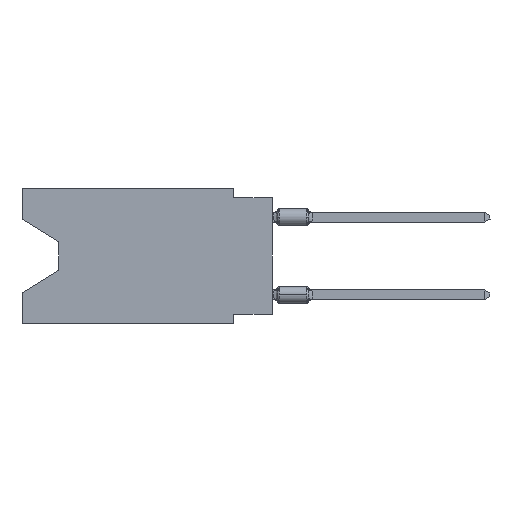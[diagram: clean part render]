
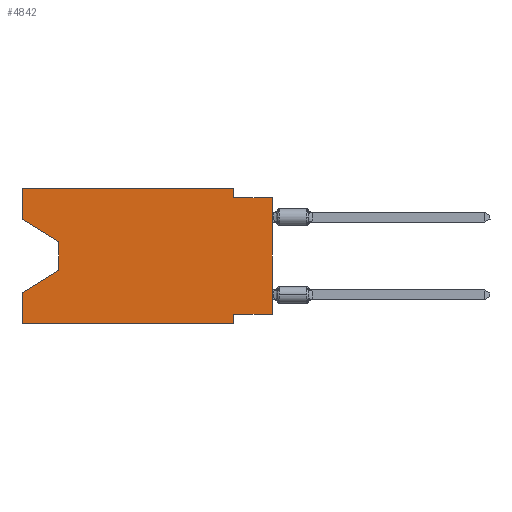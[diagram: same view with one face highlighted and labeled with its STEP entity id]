
A CAD part, left-side view. The second image highlights one B-rep face of the part: STEP entity #4842.
In plain terms, the highlighted planar face has unit normal (-1, 0, 0).
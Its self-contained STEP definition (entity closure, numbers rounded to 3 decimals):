
#241 = CARTESIAN_POINT ( 'NONE',  ( 0., 13.97, -3.505 ) ) ;
#1498 = EDGE_CURVE ( 'NONE', #16888, #11279, #6890, .T. ) ;
#1692 = DIRECTION ( 'NONE',  ( 0., 0., 1. ) ) ;
#2152 = VECTOR ( 'NONE', #27489, 1000. ) ;
#2357 = FACE_OUTER_BOUND ( 'NONE', #19299, .T. ) ;
#2875 = EDGE_CURVE ( 'NONE', #22233, #11279, #8806, .T. ) ;
#3012 = CARTESIAN_POINT ( 'NONE',  ( 0., 2.54, 0. ) ) ;
#3513 = VERTEX_POINT ( 'NONE', #21518 ) ;
#3789 = CARTESIAN_POINT ( 'NONE',  ( 0., 16.383, 0. ) ) ;
#3862 = EDGE_CURVE ( 'NONE', #16888, #35557, #32718, .T. ) ;
#3987 = DIRECTION ( 'NONE',  ( 0., 0., 1. ) ) ;
#4747 = ORIENTED_EDGE ( 'NONE', *, *, #31451, .F. ) ;
#4842 = ADVANCED_FACE ( 'NONE', ( #2357 ), #22465, .F. ) ;
#4987 = ORIENTED_EDGE ( 'NONE', *, *, #8516, .F. ) ;
#5757 = CARTESIAN_POINT ( 'NONE',  ( 0., 13.97, -3.505 ) ) ;
#6108 = DIRECTION ( 'NONE',  ( 0., 0., -1. ) ) ;
#6248 = EDGE_CURVE ( 'NONE', #24653, #28979, #10407, .T. ) ;
#6860 = ORIENTED_EDGE ( 'NONE', *, *, #25004, .T. ) ;
#6890 = LINE ( 'NONE', #21964, #22662 ) ;
#7233 = CARTESIAN_POINT ( 'NONE',  ( 0., 0., -0.635 ) ) ;
#8295 = LINE ( 'NONE', #31710, #23597 ) ;
#8516 = EDGE_CURVE ( 'NONE', #23268, #36215, #9499, .T. ) ;
#8806 = LINE ( 'NONE', #22407, #21508 ) ;
#9112 = ORIENTED_EDGE ( 'NONE', *, *, #30704, .F. ) ;
#9477 = DIRECTION ( 'NONE',  ( 0., 1., 0. ) ) ;
#9499 = LINE ( 'NONE', #21122, #2152 ) ;
#10407 = LINE ( 'NONE', #16976, #26755 ) ;
#10529 = EDGE_CURVE ( 'NONE', #18770, #3513, #32265, .T. ) ;
#10839 = LINE ( 'NONE', #26115, #38145 ) ;
#11279 = VERTEX_POINT ( 'NONE', #7233 ) ;
#12100 = CARTESIAN_POINT ( 'NONE',  ( 0., 16.383, -8.89 ) ) ;
#12760 = CARTESIAN_POINT ( 'NONE',  ( 0., 2.54, 0. ) ) ;
#13883 = CARTESIAN_POINT ( 'NONE',  ( 0., 13.97, -5.385 ) ) ;
#14752 = AXIS2_PLACEMENT_3D ( 'NONE', #16874, #34483, #29233 ) ;
#14763 = CARTESIAN_POINT ( 'NONE',  ( 0., 16.383, -6.852 ) ) ;
#15538 = ORIENTED_EDGE ( 'NONE', *, *, #6248, .F. ) ;
#16063 = ORIENTED_EDGE ( 'NONE', *, *, #3862, .F. ) ;
#16257 = VECTOR ( 'NONE', #28781, 1000. ) ;
#16424 = DIRECTION ( 'NONE',  ( 0., -1., 0. ) ) ;
#16785 = LINE ( 'NONE', #28576, #37239 ) ;
#16874 = CARTESIAN_POINT ( 'NONE',  ( 0., 16.383, 0. ) ) ;
#16888 = VERTEX_POINT ( 'NONE', #37113 ) ;
#16976 = CARTESIAN_POINT ( 'NONE',  ( 0., 16.383, 0. ) ) ;
#17051 = ORIENTED_EDGE ( 'NONE', *, *, #1498, .T. ) ;
#17569 = DIRECTION ( 'NONE',  ( 0., 0., -1. ) ) ;
#17854 = ORIENTED_EDGE ( 'NONE', *, *, #26642, .T. ) ;
#18095 = CARTESIAN_POINT ( 'NONE',  ( 0., 16.383, -2.038 ) ) ;
#18310 = ORIENTED_EDGE ( 'NONE', *, *, #29201, .T. ) ;
#18395 = VECTOR ( 'NONE', #9477, 1000. ) ;
#18770 = VERTEX_POINT ( 'NONE', #241 ) ;
#19299 = EDGE_LOOP ( 'NONE', ( #6860, #29325, #17854, #15538, #18310, #4747, #16063, #17051, #35981, #9112, #4987, #27794 ) ) ;
#21122 = CARTESIAN_POINT ( 'NONE',  ( 0., 16.383, 0. ) ) ;
#21472 = VERTEX_POINT ( 'NONE', #29192 ) ;
#21508 = VECTOR ( 'NONE', #16424, 1000. ) ;
#21518 = CARTESIAN_POINT ( 'NONE',  ( 0., 13.97, -5.385 ) ) ;
#21730 = EDGE_CURVE ( 'NONE', #37658, #23268, #16785, .T. ) ;
#21964 = CARTESIAN_POINT ( 'NONE',  ( 0., 0., 0. ) ) ;
#22233 = VERTEX_POINT ( 'NONE', #23081 ) ;
#22407 = CARTESIAN_POINT ( 'NONE',  ( 0., 0., -0.635 ) ) ;
#22430 = DIRECTION ( 'NONE',  ( 0., -0.855, -0.519 ) ) ;
#22465 = PLANE ( 'NONE',  #14752 ) ;
#22662 = VECTOR ( 'NONE', #3987, 1000. ) ;
#23081 = CARTESIAN_POINT ( 'NONE',  ( 0., 2.54, -0.635 ) ) ;
#23268 = VERTEX_POINT ( 'NONE', #3789 ) ;
#23597 = VECTOR ( 'NONE', #22430, 1000. ) ;
#24364 = LINE ( 'NONE', #12760, #31333 ) ;
#24653 = VERTEX_POINT ( 'NONE', #12100 ) ;
#25004 = EDGE_CURVE ( 'NONE', #37658, #18770, #8295, .T. ) ;
#26115 = CARTESIAN_POINT ( 'NONE',  ( 0., 16.383, -8.89 ) ) ;
#26642 = EDGE_CURVE ( 'NONE', #3513, #28979, #37125, .T. ) ;
#26755 = VECTOR ( 'NONE', #37302, 1000. ) ;
#27140 = CARTESIAN_POINT ( 'NONE',  ( 0., 2.54, -8.255 ) ) ;
#27489 = DIRECTION ( 'NONE',  ( 0., -1., 0. ) ) ;
#27794 = ORIENTED_EDGE ( 'NONE', *, *, #21730, .F. ) ;
#28576 = CARTESIAN_POINT ( 'NONE',  ( 0., 16.383, 0. ) ) ;
#28781 = DIRECTION ( 'NONE',  ( 0., 0.855, -0.519 ) ) ;
#28979 = VERTEX_POINT ( 'NONE', #14763 ) ;
#29084 = VECTOR ( 'NONE', #17569, 1000. ) ;
#29192 = CARTESIAN_POINT ( 'NONE',  ( 0., 2.54, -8.89 ) ) ;
#29201 = EDGE_CURVE ( 'NONE', #24653, #21472, #10839, .T. ) ;
#29233 = DIRECTION ( 'NONE',  ( 0., 0., -1. ) ) ;
#29325 = ORIENTED_EDGE ( 'NONE', *, *, #10529, .T. ) ;
#30119 = VECTOR ( 'NONE', #6108, 1000. ) ;
#30704 = EDGE_CURVE ( 'NONE', #36215, #22233, #24364, .T. ) ;
#30941 = DIRECTION ( 'NONE',  ( 0., 0., -1. ) ) ;
#31333 = VECTOR ( 'NONE', #30941, 1000. ) ;
#31451 = EDGE_CURVE ( 'NONE', #35557, #21472, #37854, .T. ) ;
#31710 = CARTESIAN_POINT ( 'NONE',  ( 0., 16.383, -2.038 ) ) ;
#32265 = LINE ( 'NONE', #5757, #29084 ) ;
#32318 = CARTESIAN_POINT ( 'NONE',  ( 0., 0., -8.255 ) ) ;
#32718 = LINE ( 'NONE', #32318, #18395 ) ;
#34463 = DIRECTION ( 'NONE',  ( 0., -1., 0. ) ) ;
#34483 = DIRECTION ( 'NONE',  ( 1., 0., 0. ) ) ;
#34947 = CARTESIAN_POINT ( 'NONE',  ( 0., 2.54, -8.89 ) ) ;
#35557 = VERTEX_POINT ( 'NONE', #27140 ) ;
#35981 = ORIENTED_EDGE ( 'NONE', *, *, #2875, .F. ) ;
#36215 = VERTEX_POINT ( 'NONE', #3012 ) ;
#37113 = CARTESIAN_POINT ( 'NONE',  ( 0., 0., -8.255 ) ) ;
#37125 = LINE ( 'NONE', #13883, #16257 ) ;
#37239 = VECTOR ( 'NONE', #1692, 1000. ) ;
#37302 = DIRECTION ( 'NONE',  ( 0., 0., 1. ) ) ;
#37658 = VERTEX_POINT ( 'NONE', #18095 ) ;
#37854 = LINE ( 'NONE', #34947, #30119 ) ;
#38145 = VECTOR ( 'NONE', #34463, 1000. ) ;
